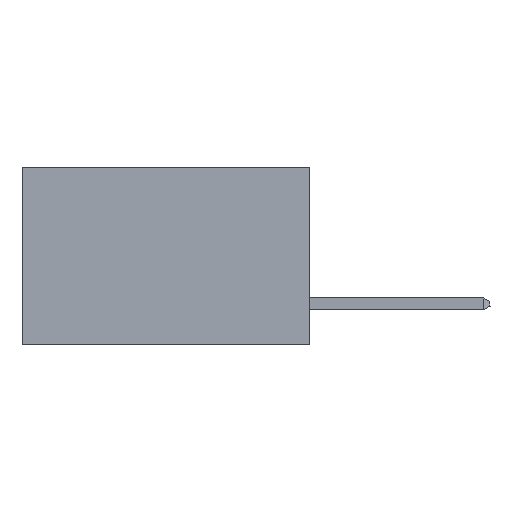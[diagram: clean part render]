
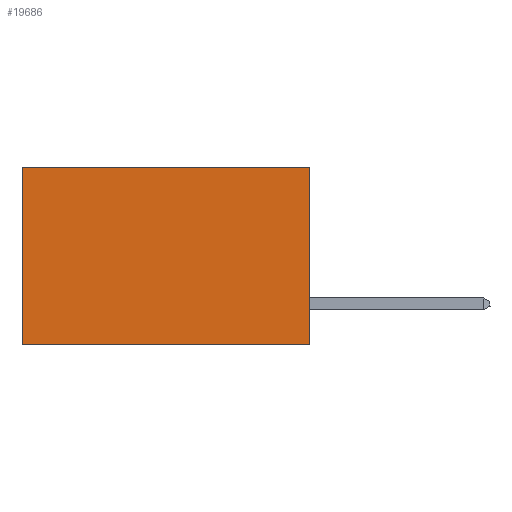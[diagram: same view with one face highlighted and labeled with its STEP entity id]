
A CAD part, left-side view. The second image highlights one B-rep face of the part: STEP entity #19686.
In plain terms, the highlighted planar face has unit normal (-1, 0, 0).
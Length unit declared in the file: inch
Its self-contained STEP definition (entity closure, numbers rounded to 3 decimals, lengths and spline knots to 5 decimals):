
#589 = EDGE_CURVE ( 'NONE', #9304, #23074, #12596, .T. ) ;
#1058 = LINE ( 'NONE', #24822, #20019 ) ;
#1325 = FACE_OUTER_BOUND ( 'NONE', #15024, .T. ) ;
#2094 = DIRECTION ( 'NONE',  ( 0., 1., 0. ) ) ;
#2792 = DIRECTION ( 'NONE',  ( 0., 0., -1. ) ) ;
#2892 = AXIS2_PLACEMENT_3D ( 'NONE', #18780, #10865, #6891 ) ;
#3932 = ORIENTED_EDGE ( 'NONE', *, *, #589, .T. ) ;
#4880 = PLANE ( 'NONE',  #2892 ) ;
#6133 = VECTOR ( 'NONE', #20910, 39.37008 ) ;
#6190 = CARTESIAN_POINT ( 'NONE',  ( 0.2875, 0., 0. ) ) ;
#6891 = DIRECTION ( 'NONE',  ( 0., 0., -1. ) ) ;
#7605 = ORIENTED_EDGE ( 'NONE', *, *, #20844, .F. ) ;
#8634 = CARTESIAN_POINT ( 'NONE',  ( 0.2875, 0., -0.37 ) ) ;
#9304 = VERTEX_POINT ( 'NONE', #25148 ) ;
#9353 = ORIENTED_EDGE ( 'NONE', *, *, #13315, .F. ) ;
#9639 = VERTEX_POINT ( 'NONE', #6190 ) ;
#10823 = VECTOR ( 'NONE', #20749, 39.37008 ) ;
#10865 = DIRECTION ( 'NONE',  ( 1., 0., 0. ) ) ;
#11410 = ORIENTED_EDGE ( 'NONE', *, *, #16795, .T. ) ;
#12596 = LINE ( 'NONE', #21084, #6133 ) ;
#12890 = VERTEX_POINT ( 'NONE', #8634 ) ;
#13315 = EDGE_CURVE ( 'NONE', #9639, #12890, #1058, .T. ) ;
#13950 = CARTESIAN_POINT ( 'NONE',  ( 0.2875, 0., -0.37 ) ) ;
#15024 = EDGE_LOOP ( 'NONE', ( #3932, #7605, #9353, #11410 ) ) ;
#15221 = LINE ( 'NONE', #13950, #18665 ) ;
#16114 = LINE ( 'NONE', #22675, #10823 ) ;
#16795 = EDGE_CURVE ( 'NONE', #9639, #9304, #16114, .T. ) ;
#18665 = VECTOR ( 'NONE', #2094, 39.37008 ) ;
#18780 = CARTESIAN_POINT ( 'NONE',  ( 0.2875, 0., 0. ) ) ;
#19686 = ADVANCED_FACE ( 'NONE', ( #1325 ), #4880, .F. ) ;
#20019 = VECTOR ( 'NONE', #2792, 39.37008 ) ;
#20749 = DIRECTION ( 'NONE',  ( 0., 1., 0. ) ) ;
#20844 = EDGE_CURVE ( 'NONE', #12890, #23074, #15221, .T. ) ;
#20910 = DIRECTION ( 'NONE',  ( 0., 0., -1. ) ) ;
#21084 = CARTESIAN_POINT ( 'NONE',  ( 0.2875, 0.6, 0. ) ) ;
#22675 = CARTESIAN_POINT ( 'NONE',  ( 0.2875, 0., 0. ) ) ;
#23074 = VERTEX_POINT ( 'NONE', #23198 ) ;
#23198 = CARTESIAN_POINT ( 'NONE',  ( 0.2875, 0.6, -0.37 ) ) ;
#24822 = CARTESIAN_POINT ( 'NONE',  ( 0.2875, 0., 0. ) ) ;
#25148 = CARTESIAN_POINT ( 'NONE',  ( 0.2875, 0.6, 0. ) ) ;
